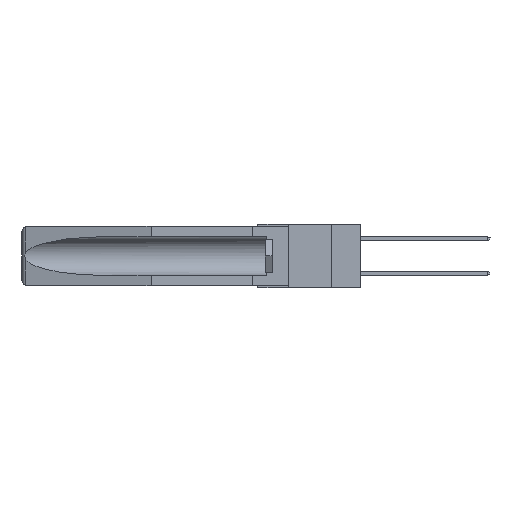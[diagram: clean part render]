
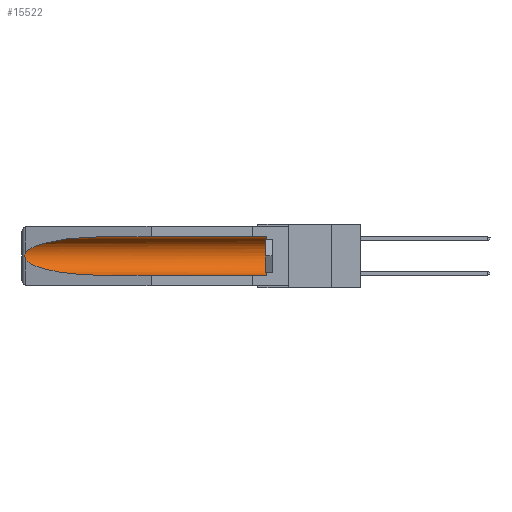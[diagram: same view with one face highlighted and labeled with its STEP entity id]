
A CAD part, left-side view. The second image highlights one B-rep face of the part: STEP entity #15522.
In plain terms, the highlighted cylindrical face has radius 2.857 mm (diameter 5.715 mm), a partial arc.
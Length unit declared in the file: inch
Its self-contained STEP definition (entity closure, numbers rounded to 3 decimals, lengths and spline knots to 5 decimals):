
#459 = CARTESIAN_POINT ( 'NONE',  ( 0.155, 1.07973, -0.059 ) ) ;
#604 = VECTOR ( 'NONE', #4503, 39.37008 ) ;
#632 = ORIENTED_EDGE ( 'NONE', *, *, #20881, .T. ) ;
#941 = CARTESIAN_POINT ( 'NONE',  ( 0.155, -0.30754, -0.1715 ) ) ;
#1233 = B_SPLINE_CURVE_WITH_KNOTS ( 'NONE', 3,
 ( #21543, #11696, #31682, #13955, #3950, #1735, #8834, #16564, #26923, #6422 ),
 .UNSPECIFIED., .F., .F.,
 ( 4, 2, 2, 2, 4 ),
 ( 0., 0.00029, 0.00058, 0.00087, 0.00117 ),
 .UNSPECIFIED. ) ;
#1735 = CARTESIAN_POINT ( 'NONE',  ( 0.2675, 1.53308, -0.17534 ) ) ;
#3291 = CARTESIAN_POINT ( 'NONE',  ( 0.155, 0.126, -0.284 ) ) ;
#3501 = EDGE_CURVE ( 'NONE', #5408, #13226, #1233, .T. ) ;
#3588 = CARTESIAN_POINT ( 'NONE',  ( 0.155, 0.126, -0.1715 ) ) ;
#3950 = CARTESIAN_POINT ( 'NONE',  ( 0.2675, 1.53308, -0.16763 ) ) ;
#4503 = DIRECTION ( 'NONE',  ( 0., 1., 0. ) ) ;
#4512 = FACE_OUTER_BOUND ( 'NONE', #32605, .T. ) ;
#4602 = CARTESIAN_POINT ( 'NONE',  ( 0.155, -0.30754, -0.059 ) ) ;
#4755 = ORIENTED_EDGE ( 'NONE', *, *, #3501, .T. ) ;
#5408 = VERTEX_POINT ( 'NONE', #10692 ) ;
#5738 = AXIS2_PLACEMENT_3D ( 'NONE', #3588, #11230, #21086 ) ;
#6422 = CARTESIAN_POINT ( 'NONE',  ( 0.26537, 1.52718, -0.19328 ) ) ;
#7209 = ORIENTED_EDGE ( 'NONE', *, *, #14944, .T. ) ;
#8044 = ORIENTED_EDGE ( 'NONE', *, *, #19605, .T. ) ;
#8321 = CARTESIAN_POINT ( 'NONE',  ( 0.155, 1.07973, -0.284 ) ) ;
#8834 = CARTESIAN_POINT ( 'NONE',  ( 0.2673, 1.53269, -0.17917 ) ) ;
#10544 = CARTESIAN_POINT ( 'NONE',  ( 0.155, 1.07973, -0.284 ) ) ;
#10692 = CARTESIAN_POINT ( 'NONE',  ( 0.26537, 1.52718, -0.14972 ) ) ;
#10881 = DIRECTION ( 'NONE',  ( 0., 0., 1. ) ) ;
#10995 = DIRECTION ( 'NONE',  ( 0., 1., 0. ) ) ;
#11230 = DIRECTION ( 'NONE',  ( 0., -1., 0. ) ) ;
#11352 = CARTESIAN_POINT ( 'NONE',  ( 0.26537, 1.52718, -0.19328 ) ) ;
#11491 = EDGE_CURVE ( 'NONE', #21945, #24417, #29156, .T. ) ;
#11696 = CARTESIAN_POINT ( 'NONE',  ( 0.26597, 1.52961, -0.15275 ) ) ;
#12012 = LINE ( 'NONE', #16609, #21138 ) ;
#13226 = VERTEX_POINT ( 'NONE', #11352 ) ;
#13955 = CARTESIAN_POINT ( 'NONE',  ( 0.2673, 1.5327, -0.16383 ) ) ;
#14554 = EDGE_CURVE ( 'NONE', #21945, #25701, #12012, .T. ) ;
#14944 = EDGE_CURVE ( 'NONE', #31614, #5408, #19733, .T. ) ;
#15513 = CYLINDRICAL_SURFACE ( 'NONE', #16161, 0.1125 ) ;
#15522 = ADVANCED_FACE ( 'NONE', ( #4512 ), #15513, .F. ) ;
#16161 = AXIS2_PLACEMENT_3D ( 'NONE', #941, #10995, #10881 ) ;
#16564 = CARTESIAN_POINT ( 'NONE',  ( 0.26655, 1.53094, -0.18657 ) ) ;
#16609 = CARTESIAN_POINT ( 'NONE',  ( 0.155, -0.30754, -0.284 ) ) ;
#17004 = CARTESIAN_POINT ( 'NONE',  ( 0.155, 1.07973, -0.059 ) ) ;
#18369 = CARTESIAN_POINT ( 'NONE',  ( 0.21114, 1.30732, -0.059 ) ) ;
#19605 = EDGE_CURVE ( 'NONE', #24417, #31614, #24217, .T. ) ;
#19650 = CARTESIAN_POINT ( 'NONE',  ( 0.155, 0.126, -0.059 ) ) ;
#19733 =( BOUNDED_CURVE ( )  B_SPLINE_CURVE ( 3, ( #459, #18369, #21035, #28420 ),
 .UNSPECIFIED., .F., .F. ) 
 B_SPLINE_CURVE_WITH_KNOTS ( ( 4, 4 ),
 ( 4.71239, 6.08839 ),
 .UNSPECIFIED. ) 
 CURVE ( )  GEOMETRIC_REPRESENTATION_ITEM ( )  RATIONAL_B_SPLINE_CURVE ( ( 1., 0.848, 0.848, 1. ) ) 
 REPRESENTATION_ITEM ( '' )  );
#20881 = EDGE_CURVE ( 'NONE', #13226, #25701, #21198, .T. ) ;
#20913 = CARTESIAN_POINT ( 'NONE',  ( 0.25451, 1.48313, -0.24835 ) ) ;
#21035 = CARTESIAN_POINT ( 'NONE',  ( 0.25451, 1.48313, -0.09465 ) ) ;
#21086 = DIRECTION ( 'NONE',  ( 0., 0., 1. ) ) ;
#21138 = VECTOR ( 'NONE', #26550, 39.37008 ) ;
#21198 =( BOUNDED_CURVE ( )  B_SPLINE_CURVE ( 3, ( #22899, #20913, #23448, #8321 ),
 .UNSPECIFIED., .F., .F. ) 
 B_SPLINE_CURVE_WITH_KNOTS ( ( 4, 4 ),
 ( 0.1948, 1.5708 ),
 .UNSPECIFIED. ) 
 CURVE ( )  GEOMETRIC_REPRESENTATION_ITEM ( )  RATIONAL_B_SPLINE_CURVE ( ( 1., 0.848, 0.848, 1. ) ) 
 REPRESENTATION_ITEM ( '' )  );
#21543 = CARTESIAN_POINT ( 'NONE',  ( 0.26537, 1.52718, -0.14972 ) ) ;
#21945 = VERTEX_POINT ( 'NONE', #3291 ) ;
#22849 = ORIENTED_EDGE ( 'NONE', *, *, #14554, .F. ) ;
#22899 = CARTESIAN_POINT ( 'NONE',  ( 0.26537, 1.52718, -0.19328 ) ) ;
#23448 = CARTESIAN_POINT ( 'NONE',  ( 0.21114, 1.30732, -0.284 ) ) ;
#24217 = LINE ( 'NONE', #4602, #604 ) ;
#24417 = VERTEX_POINT ( 'NONE', #19650 ) ;
#25701 = VERTEX_POINT ( 'NONE', #10544 ) ;
#26550 = DIRECTION ( 'NONE',  ( 0., 1., 0. ) ) ;
#26696 = ORIENTED_EDGE ( 'NONE', *, *, #11491, .T. ) ;
#26923 = CARTESIAN_POINT ( 'NONE',  ( 0.26597, 1.5296, -0.19026 ) ) ;
#28420 = CARTESIAN_POINT ( 'NONE',  ( 0.26537, 1.52718, -0.14972 ) ) ;
#29156 = CIRCLE ( 'NONE', #5738, 0.1125 ) ;
#31614 = VERTEX_POINT ( 'NONE', #17004 ) ;
#31682 = CARTESIAN_POINT ( 'NONE',  ( 0.26654, 1.53092, -0.15636 ) ) ;
#32605 = EDGE_LOOP ( 'NONE', ( #7209, #4755, #632, #22849, #26696, #8044 ) ) ;
